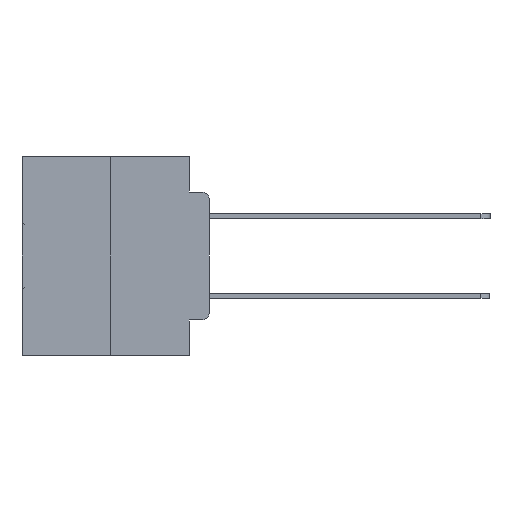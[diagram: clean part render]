
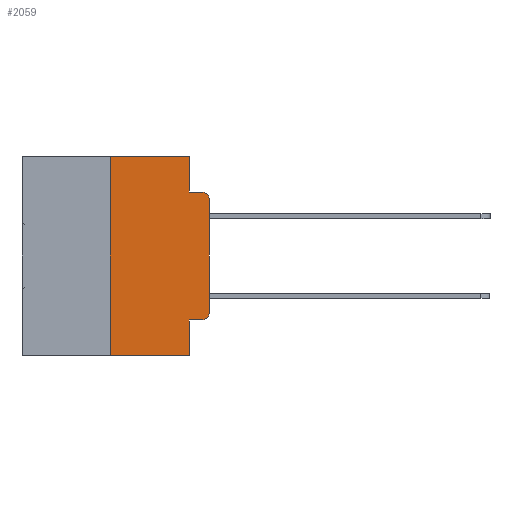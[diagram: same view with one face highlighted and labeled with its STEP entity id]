
A CAD part, left-side view. The second image highlights one B-rep face of the part: STEP entity #2059.
In plain terms, the highlighted planar face has unit normal (-1, 0, 0).
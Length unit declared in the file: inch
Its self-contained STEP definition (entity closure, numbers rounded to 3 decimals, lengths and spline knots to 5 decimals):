
#26 = LINE ( 'NONE', #5323, #20343 ) ;
#744 = ORIENTED_EDGE ( 'NONE', *, *, #1739, .T. ) ;
#1268 = CARTESIAN_POINT ( 'NONE',  ( 0., 0., -0.1085 ) ) ;
#1739 = EDGE_CURVE ( 'NONE', #16510, #9732, #15869, .T. ) ;
#1970 = LINE ( 'NONE', #27265, #28998 ) ;
#1991 = ORIENTED_EDGE ( 'NONE', *, *, #20124, .F. ) ;
#2059 = ADVANCED_FACE ( 'NONE', ( #12491 ), #14781, .F. ) ;
#2617 = CARTESIAN_POINT ( 'NONE',  ( 0., 0.473, -0.5 ) ) ;
#2676 = CARTESIAN_POINT ( 'NONE',  ( 0., 0.051, -0.0885 ) ) ;
#2770 = CARTESIAN_POINT ( 'NONE',  ( 0., 0.25, 0. ) ) ;
#3251 = VERTEX_POINT ( 'NONE', #25121 ) ;
#3397 = CARTESIAN_POINT ( 'NONE',  ( 0., 0.02, -0.0885 ) ) ;
#3716 = CIRCLE ( 'NONE', #19076, 0.02 ) ;
#3732 = VERTEX_POINT ( 'NONE', #21163 ) ;
#3973 = LINE ( 'NONE', #15258, #24072 ) ;
#5117 = EDGE_CURVE ( 'NONE', #18397, #7394, #13967, .T. ) ;
#5323 = CARTESIAN_POINT ( 'NONE',  ( 0., 0., 0. ) ) ;
#5732 = DIRECTION ( 'NONE',  ( 0., 0., -1. ) ) ;
#5937 = LINE ( 'NONE', #30137, #25953 ) ;
#6366 = CARTESIAN_POINT ( 'NONE',  ( 0., 0.051, -0.4115 ) ) ;
#7394 = VERTEX_POINT ( 'NONE', #9006 ) ;
#7563 = CARTESIAN_POINT ( 'NONE',  ( 0., 0.25, -0.5 ) ) ;
#7834 = ORIENTED_EDGE ( 'NONE', *, *, #8436, .T. ) ;
#8436 = EDGE_CURVE ( 'NONE', #3732, #31509, #26, .T. ) ;
#9006 = CARTESIAN_POINT ( 'NONE',  ( 0., 0.051, -0.5 ) ) ;
#9071 = DIRECTION ( 'NONE',  ( 0., -1., 0. ) ) ;
#9105 = ORIENTED_EDGE ( 'NONE', *, *, #5117, .T. ) ;
#9441 = DIRECTION ( 'NONE',  ( -1., 0., 0. ) ) ;
#9596 = EDGE_CURVE ( 'NONE', #31509, #10748, #27491, .T. ) ;
#9732 = VERTEX_POINT ( 'NONE', #28071 ) ;
#10352 = DIRECTION ( 'NONE',  ( -1., 0., 0. ) ) ;
#10748 = VERTEX_POINT ( 'NONE', #3397 ) ;
#11209 = AXIS2_PLACEMENT_3D ( 'NONE', #14716, #14755, #5732 ) ;
#11270 = VERTEX_POINT ( 'NONE', #2770 ) ;
#12491 = FACE_OUTER_BOUND ( 'NONE', #18640, .T. ) ;
#12621 = DIRECTION ( 'NONE',  ( 0., 0., -1. ) ) ;
#13136 = VECTOR ( 'NONE', #30820, 39.37008 ) ;
#13213 = ORIENTED_EDGE ( 'NONE', *, *, #9596, .T. ) ;
#13967 = LINE ( 'NONE', #2617, #13136 ) ;
#14488 = ORIENTED_EDGE ( 'NONE', *, *, #14898, .F. ) ;
#14519 = ORIENTED_EDGE ( 'NONE', *, *, #30464, .T. ) ;
#14702 = AXIS2_PLACEMENT_3D ( 'NONE', #25030, #9441, #27616 ) ;
#14716 = CARTESIAN_POINT ( 'NONE',  ( 0., 0.473, 0. ) ) ;
#14755 = DIRECTION ( 'NONE',  ( 1., 0., 0. ) ) ;
#14781 = PLANE ( 'NONE',  #11209 ) ;
#14898 = EDGE_CURVE ( 'NONE', #3251, #23749, #3973, .T. ) ;
#15258 = CARTESIAN_POINT ( 'NONE',  ( 0., 0.051, 0. ) ) ;
#15696 = CARTESIAN_POINT ( 'NONE',  ( 0., 0.051, -0.4115 ) ) ;
#15869 = LINE ( 'NONE', #15696, #28803 ) ;
#16510 = VERTEX_POINT ( 'NONE', #6366 ) ;
#18397 = VERTEX_POINT ( 'NONE', #7563 ) ;
#18609 = ORIENTED_EDGE ( 'NONE', *, *, #23550, .F. ) ;
#18640 = EDGE_LOOP ( 'NONE', ( #7834, #13213, #27408, #14488, #1991, #18609, #9105, #22606, #744, #14519 ) ) ;
#19076 = AXIS2_PLACEMENT_3D ( 'NONE', #25908, #10352, #28495 ) ;
#20124 = EDGE_CURVE ( 'NONE', #11270, #3251, #1970, .T. ) ;
#20343 = VECTOR ( 'NONE', #21063, 39.37008 ) ;
#20460 = DIRECTION ( 'NONE',  ( 0., -1., 0. ) ) ;
#21063 = DIRECTION ( 'NONE',  ( 0., 0., 1. ) ) ;
#21163 = CARTESIAN_POINT ( 'NONE',  ( 0., 0., -0.3915 ) ) ;
#21833 = EDGE_CURVE ( 'NONE', #23749, #10748, #31298, .T. ) ;
#22606 = ORIENTED_EDGE ( 'NONE', *, *, #28727, .F. ) ;
#23151 = LINE ( 'NONE', #23842, #29170 ) ;
#23550 = EDGE_CURVE ( 'NONE', #18397, #11270, #5937, .T. ) ;
#23749 = VERTEX_POINT ( 'NONE', #2676 ) ;
#23842 = CARTESIAN_POINT ( 'NONE',  ( 0., 0.051, 0. ) ) ;
#24072 = VECTOR ( 'NONE', #12621, 39.37008 ) ;
#24961 = DIRECTION ( 'NONE',  ( 0., 0., 1. ) ) ;
#25030 = CARTESIAN_POINT ( 'NONE',  ( 0., 0.02, -0.1085 ) ) ;
#25121 = CARTESIAN_POINT ( 'NONE',  ( 0., 0.051, 0. ) ) ;
#25908 = CARTESIAN_POINT ( 'NONE',  ( 0., 0.02, -0.3915 ) ) ;
#25953 = VECTOR ( 'NONE', #24961, 39.37008 ) ;
#27265 = CARTESIAN_POINT ( 'NONE',  ( 0., 0.473, 0. ) ) ;
#27408 = ORIENTED_EDGE ( 'NONE', *, *, #21833, .F. ) ;
#27491 = CIRCLE ( 'NONE', #14702, 0.02 ) ;
#27616 = DIRECTION ( 'NONE',  ( 0., 0., -1. ) ) ;
#28071 = CARTESIAN_POINT ( 'NONE',  ( 0., 0.02, -0.4115 ) ) ;
#28495 = DIRECTION ( 'NONE',  ( 0., 0., -1. ) ) ;
#28727 = EDGE_CURVE ( 'NONE', #16510, #7394, #23151, .T. ) ;
#28803 = VECTOR ( 'NONE', #33448, 39.37008 ) ;
#28998 = VECTOR ( 'NONE', #9071, 39.37008 ) ;
#29030 = DIRECTION ( 'NONE',  ( 0., 0., -1. ) ) ;
#29170 = VECTOR ( 'NONE', #29030, 39.37008 ) ;
#30137 = CARTESIAN_POINT ( 'NONE',  ( 0., 0.25, 0. ) ) ;
#30464 = EDGE_CURVE ( 'NONE', #9732, #3732, #3716, .T. ) ;
#30509 = VECTOR ( 'NONE', #20460, 39.37008 ) ;
#30679 = CARTESIAN_POINT ( 'NONE',  ( 0., 0.051, -0.0885 ) ) ;
#30820 = DIRECTION ( 'NONE',  ( 0., -1., 0. ) ) ;
#31298 = LINE ( 'NONE', #30679, #30509 ) ;
#31509 = VERTEX_POINT ( 'NONE', #1268 ) ;
#33448 = DIRECTION ( 'NONE',  ( 0., -1., 0. ) ) ;
